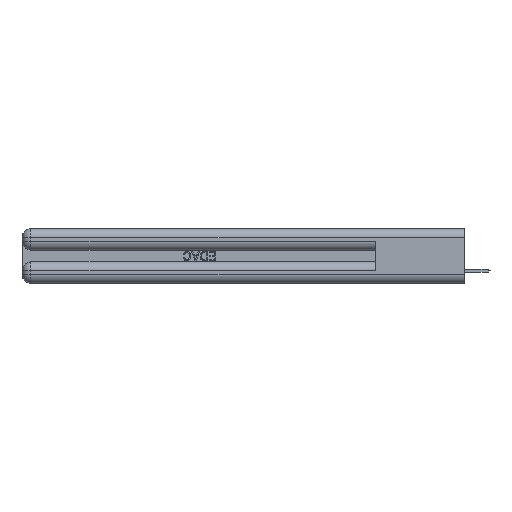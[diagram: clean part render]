
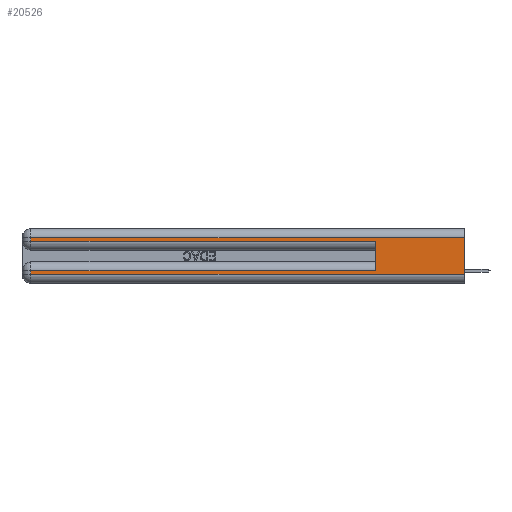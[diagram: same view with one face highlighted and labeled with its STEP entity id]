
A CAD part, left-side view. The second image highlights one B-rep face of the part: STEP entity #20526.
In plain terms, the highlighted planar face has unit normal (-1, 0, 0).
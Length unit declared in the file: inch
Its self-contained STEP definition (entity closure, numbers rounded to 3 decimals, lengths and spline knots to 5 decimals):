
#2 = ORIENTED_EDGE ( 'NONE', *, *, #15714, .T. ) ;
#804 = ORIENTED_EDGE ( 'NONE', *, *, #41985, .T. ) ;
#849 = CARTESIAN_POINT ( 'NONE',  ( 0., 0.6, 0.085 ) ) ;
#2142 = PLANE ( 'NONE',  #29946 ) ;
#4744 = CARTESIAN_POINT ( 'NONE',  ( 0., 0.6, 0.145 ) ) ;
#5022 = DIRECTION ( 'NONE',  ( 0., -1., 0. ) ) ;
#5193 = DIRECTION ( 'NONE',  ( 0., -1., 0. ) ) ;
#5392 = VECTOR ( 'NONE', #27343, 39.37008 ) ;
#5975 = DIRECTION ( 'NONE',  ( 0., 0., -1. ) ) ;
#6414 = EDGE_CURVE ( 'NONE', #23449, #45011, #44067, .T. ) ;
#7063 = LINE ( 'NONE', #4744, #33156 ) ;
#7626 = LINE ( 'NONE', #24228, #5392 ) ;
#7776 = CARTESIAN_POINT ( 'NONE',  ( 0., 0., 0.06 ) ) ;
#11097 = LINE ( 'NONE', #19967, #16129 ) ;
#12083 = CARTESIAN_POINT ( 'NONE',  ( 0., 0., 0.06 ) ) ;
#13377 = VERTEX_POINT ( 'NONE', #34697 ) ;
#13990 = CARTESIAN_POINT ( 'NONE',  ( 0., 2.94, 0.06 ) ) ;
#14316 = VERTEX_POINT ( 'NONE', #32737 ) ;
#15032 = VECTOR ( 'NONE', #15138, 39.37008 ) ;
#15138 = DIRECTION ( 'NONE',  ( 0., 1., 0. ) ) ;
#15714 = EDGE_CURVE ( 'NONE', #45583, #26414, #24281, .T. ) ;
#16004 = CARTESIAN_POINT ( 'NONE',  ( 0., 0., 0.285 ) ) ;
#16129 = VECTOR ( 'NONE', #37953, 39.37008 ) ;
#16276 = ORIENTED_EDGE ( 'NONE', *, *, #32682, .T. ) ;
#16598 = DIRECTION ( 'NONE',  ( 1., 0., 0. ) ) ;
#18750 = CARTESIAN_POINT ( 'NONE',  ( 0., 0., 0.31 ) ) ;
#19195 = VECTOR ( 'NONE', #40588, 39.37008 ) ;
#19233 = ORIENTED_EDGE ( 'NONE', *, *, #6414, .T. ) ;
#19262 = FACE_OUTER_BOUND ( 'NONE', #30708, .T. ) ;
#19967 = CARTESIAN_POINT ( 'NONE',  ( 0., 2.94, 0.37 ) ) ;
#20526 = ADVANCED_FACE ( 'NONE', ( #19262 ), #2142, .F. ) ;
#23449 = VERTEX_POINT ( 'NONE', #13990 ) ;
#23478 = ORIENTED_EDGE ( 'NONE', *, *, #39483, .T. ) ;
#23968 = VECTOR ( 'NONE', #5022, 39.37008 ) ;
#24151 = VECTOR ( 'NONE', #5193, 39.37008 ) ;
#24228 = CARTESIAN_POINT ( 'NONE',  ( 0., 0., 0.37 ) ) ;
#24281 = LINE ( 'NONE', #34034, #38741 ) ;
#24993 = ORIENTED_EDGE ( 'NONE', *, *, #43911, .F. ) ;
#26376 = LINE ( 'NONE', #33721, #19195 ) ;
#26414 = VERTEX_POINT ( 'NONE', #42773 ) ;
#27343 = DIRECTION ( 'NONE',  ( 0., 0., -1. ) ) ;
#29485 = DIRECTION ( 'NONE',  ( 0., 0., 1. ) ) ;
#29692 = ORIENTED_EDGE ( 'NONE', *, *, #42385, .T. ) ;
#29946 = AXIS2_PLACEMENT_3D ( 'NONE', #38876, #16598, #5975 ) ;
#30708 = EDGE_LOOP ( 'NONE', ( #34934, #804, #29692, #16276, #24993, #2, #23478, #19233 ) ) ;
#32682 = EDGE_CURVE ( 'NONE', #14316, #45626, #33015, .T. ) ;
#32737 = CARTESIAN_POINT ( 'NONE',  ( 0., 2.94, 0.285 ) ) ;
#33015 = LINE ( 'NONE', #16004, #24151 ) ;
#33156 = VECTOR ( 'NONE', #29485, 39.37008 ) ;
#33721 = CARTESIAN_POINT ( 'NONE',  ( 0., 2.94, 0.37 ) ) ;
#34034 = CARTESIAN_POINT ( 'NONE',  ( 0., 0., 0.085 ) ) ;
#34697 = CARTESIAN_POINT ( 'NONE',  ( 0., 2.94, 0.31 ) ) ;
#34934 = ORIENTED_EDGE ( 'NONE', *, *, #36608, .F. ) ;
#36059 = CARTESIAN_POINT ( 'NONE',  ( 0., 0., 0.31 ) ) ;
#36174 = VERTEX_POINT ( 'NONE', #36059 ) ;
#36608 = EDGE_CURVE ( 'NONE', #36174, #45011, #7626, .T. ) ;
#37953 = DIRECTION ( 'NONE',  ( 0., 0., -1. ) ) ;
#38741 = VECTOR ( 'NONE', #44530, 39.37008 ) ;
#38876 = CARTESIAN_POINT ( 'NONE',  ( 0., 0., 0.37 ) ) ;
#39483 = EDGE_CURVE ( 'NONE', #26414, #23449, #26376, .T. ) ;
#39771 = CARTESIAN_POINT ( 'NONE',  ( 0., 0.6, 0.285 ) ) ;
#40588 = DIRECTION ( 'NONE',  ( 0., 0., -1. ) ) ;
#41985 = EDGE_CURVE ( 'NONE', #36174, #13377, #42308, .T. ) ;
#42308 = LINE ( 'NONE', #18750, #15032 ) ;
#42385 = EDGE_CURVE ( 'NONE', #13377, #14316, #11097, .T. ) ;
#42773 = CARTESIAN_POINT ( 'NONE',  ( 0., 2.94, 0.085 ) ) ;
#43911 = EDGE_CURVE ( 'NONE', #45583, #45626, #7063, .T. ) ;
#44067 = LINE ( 'NONE', #12083, #23968 ) ;
#44530 = DIRECTION ( 'NONE',  ( 0., 1., 0. ) ) ;
#45011 = VERTEX_POINT ( 'NONE', #7776 ) ;
#45583 = VERTEX_POINT ( 'NONE', #849 ) ;
#45626 = VERTEX_POINT ( 'NONE', #39771 ) ;
